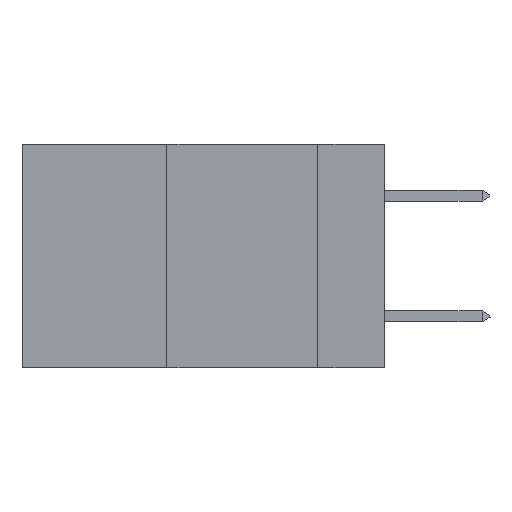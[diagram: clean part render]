
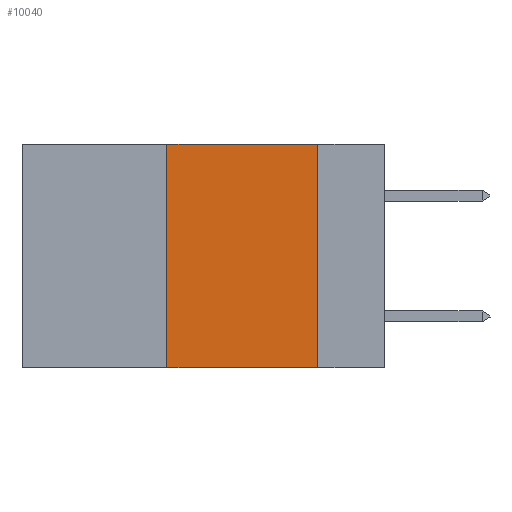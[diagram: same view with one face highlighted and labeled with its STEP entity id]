
A CAD part, left-side view. The second image highlights one B-rep face of the part: STEP entity #10040.
In plain terms, the highlighted planar face has unit normal (-1, 0, 0).
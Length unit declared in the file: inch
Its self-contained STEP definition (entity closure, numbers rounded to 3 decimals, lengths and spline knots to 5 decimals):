
#96 = ORIENTED_EDGE ( 'NONE', *, *, #21703, .F. ) ;
#367 = DIRECTION ( 'NONE',  ( 0., 0., -1. ) ) ;
#795 = AXIS2_PLACEMENT_3D ( 'NONE', #4231, #12757, #367 ) ;
#1064 = LINE ( 'NONE', #15868, #13039 ) ;
#1907 = LINE ( 'NONE', #24520, #22532 ) ;
#2501 = CARTESIAN_POINT ( 'NONE',  ( 0., 0.6, 0. ) ) ;
#2537 = CARTESIAN_POINT ( 'NONE',  ( 0., 0.36, 0. ) ) ;
#2613 = VERTEX_POINT ( 'NONE', #2537 ) ;
#2790 = CARTESIAN_POINT ( 'NONE',  ( 0., 0.36, 0. ) ) ;
#4033 = ORIENTED_EDGE ( 'NONE', *, *, #26063, .T. ) ;
#4231 = CARTESIAN_POINT ( 'NONE',  ( 0., 0.6, 0. ) ) ;
#6769 = EDGE_CURVE ( 'NONE', #20994, #22101, #1907, .T. ) ;
#8401 = CARTESIAN_POINT ( 'NONE',  ( 0., 0.11, -0.37 ) ) ;
#10040 = ADVANCED_FACE ( 'NONE', ( #16570 ), #25068, .F. ) ;
#10050 = EDGE_CURVE ( 'NONE', #2613, #20994, #17571, .T. ) ;
#12203 = DIRECTION ( 'NONE',  ( 0., 0., -1. ) ) ;
#12757 = DIRECTION ( 'NONE',  ( 1., 0., 0. ) ) ;
#13039 = VECTOR ( 'NONE', #22030, 39.37008 ) ;
#15868 = CARTESIAN_POINT ( 'NONE',  ( 0., 0.6, -0.37 ) ) ;
#15888 = VERTEX_POINT ( 'NONE', #22679 ) ;
#16570 = FACE_OUTER_BOUND ( 'NONE', #21002, .T. ) ;
#16893 = DIRECTION ( 'NONE',  ( 0., -1., 0. ) ) ;
#17037 = CARTESIAN_POINT ( 'NONE',  ( 0., 0.11, 0. ) ) ;
#17571 = LINE ( 'NONE', #2501, #26583 ) ;
#20595 = ORIENTED_EDGE ( 'NONE', *, *, #6769, .F. ) ;
#20994 = VERTEX_POINT ( 'NONE', #17037 ) ;
#21002 = EDGE_LOOP ( 'NONE', ( #20595, #21662, #96, #4033 ) ) ;
#21662 = ORIENTED_EDGE ( 'NONE', *, *, #10050, .F. ) ;
#21703 = EDGE_CURVE ( 'NONE', #15888, #2613, #25479, .T. ) ;
#22030 = DIRECTION ( 'NONE',  ( 0., -1., 0. ) ) ;
#22101 = VERTEX_POINT ( 'NONE', #8401 ) ;
#22532 = VECTOR ( 'NONE', #12203, 39.37008 ) ;
#22679 = CARTESIAN_POINT ( 'NONE',  ( 0., 0.36, -0.37 ) ) ;
#23376 = DIRECTION ( 'NONE',  ( 0., 0., 1. ) ) ;
#24520 = CARTESIAN_POINT ( 'NONE',  ( 0., 0.11, 0. ) ) ;
#25068 = PLANE ( 'NONE',  #795 ) ;
#25479 = LINE ( 'NONE', #2790, #26466 ) ;
#26063 = EDGE_CURVE ( 'NONE', #15888, #22101, #1064, .T. ) ;
#26466 = VECTOR ( 'NONE', #23376, 39.37008 ) ;
#26583 = VECTOR ( 'NONE', #16893, 39.37008 ) ;
